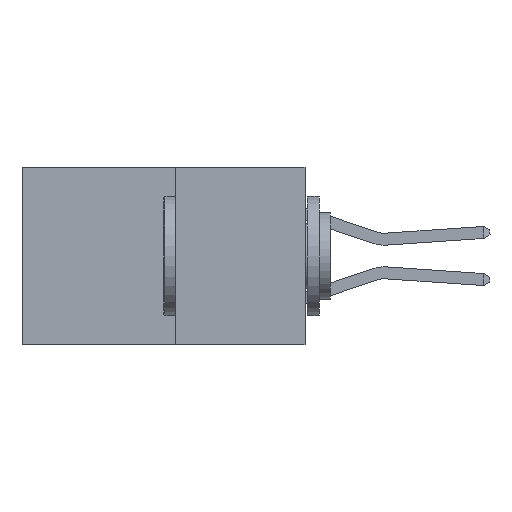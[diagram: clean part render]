
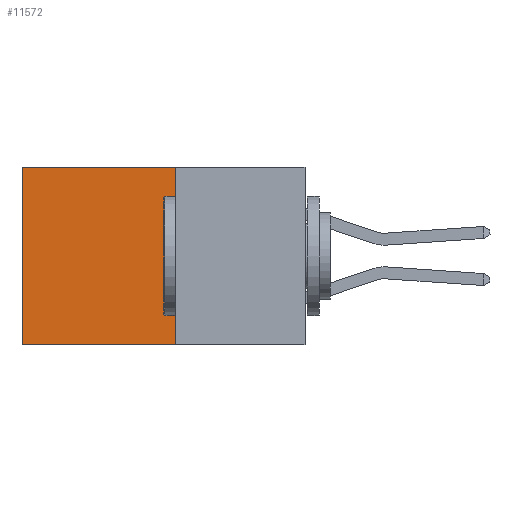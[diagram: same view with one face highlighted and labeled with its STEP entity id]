
A CAD part, left-side view. The second image highlights one B-rep face of the part: STEP entity #11572.
In plain terms, the highlighted planar face has unit normal (-1, 0, 0).
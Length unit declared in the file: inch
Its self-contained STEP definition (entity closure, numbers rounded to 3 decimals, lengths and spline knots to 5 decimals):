
#78 = VERTEX_POINT ( 'NONE', #3665 ) ;
#897 = CARTESIAN_POINT ( 'NONE',  ( 0.277, 0.27, 0. ) ) ;
#2368 = AXIS2_PLACEMENT_3D ( 'NONE', #15772, #6778, #19437 ) ;
#2902 = DIRECTION ( 'NONE',  ( 0., 0., -1. ) ) ;
#3665 = CARTESIAN_POINT ( 'NONE',  ( 0.277, 0.27, -0.37 ) ) ;
#3855 = LINE ( 'NONE', #17433, #17762 ) ;
#4111 = CARTESIAN_POINT ( 'NONE',  ( 0.277, 0.27, -0.37 ) ) ;
#4537 = CARTESIAN_POINT ( 'NONE',  ( 0.277, 0.59, -0.37 ) ) ;
#4539 = VECTOR ( 'NONE', #16781, 39.37008 ) ;
#4822 = LINE ( 'NONE', #22801, #9086 ) ;
#5117 = LINE ( 'NONE', #4111, #4539 ) ;
#6778 = DIRECTION ( 'NONE',  ( 1., 0., 0. ) ) ;
#8718 = VECTOR ( 'NONE', #19050, 39.37008 ) ;
#9086 = VECTOR ( 'NONE', #2902, 39.37008 ) ;
#9468 = EDGE_CURVE ( 'NONE', #78, #17391, #3855, .T. ) ;
#10174 = VERTEX_POINT ( 'NONE', #15640 ) ;
#11474 = VERTEX_POINT ( 'NONE', #897 ) ;
#11572 = ADVANCED_FACE ( 'NONE', ( #11981 ), #15694, .F. ) ;
#11981 = FACE_OUTER_BOUND ( 'NONE', #17147, .T. ) ;
#13414 = ORIENTED_EDGE ( 'NONE', *, *, #13504, .T. ) ;
#13504 = EDGE_CURVE ( 'NONE', #11474, #10174, #23144, .T. ) ;
#13761 = DIRECTION ( 'NONE',  ( 0., 1., 0. ) ) ;
#15530 = ORIENTED_EDGE ( 'NONE', *, *, #9468, .F. ) ;
#15640 = CARTESIAN_POINT ( 'NONE',  ( 0.277, 0.59, 0. ) ) ;
#15694 = PLANE ( 'NONE',  #2368 ) ;
#15772 = CARTESIAN_POINT ( 'NONE',  ( 0.277, 0.27, -0.37 ) ) ;
#16781 = DIRECTION ( 'NONE',  ( 0., 0., -1. ) ) ;
#17147 = EDGE_LOOP ( 'NONE', ( #18740, #15530, #20108, #13414 ) ) ;
#17391 = VERTEX_POINT ( 'NONE', #4537 ) ;
#17433 = CARTESIAN_POINT ( 'NONE',  ( 0.277, 0.27, -0.37 ) ) ;
#17762 = VECTOR ( 'NONE', #13761, 39.37008 ) ;
#17912 = EDGE_CURVE ( 'NONE', #11474, #78, #5117, .T. ) ;
#18163 = EDGE_CURVE ( 'NONE', #10174, #17391, #4822, .T. ) ;
#18740 = ORIENTED_EDGE ( 'NONE', *, *, #18163, .T. ) ;
#19050 = DIRECTION ( 'NONE',  ( 0., 1., 0. ) ) ;
#19437 = DIRECTION ( 'NONE',  ( 0., 0., -1. ) ) ;
#20108 = ORIENTED_EDGE ( 'NONE', *, *, #17912, .F. ) ;
#22671 = CARTESIAN_POINT ( 'NONE',  ( 0.277, 0.27, 0. ) ) ;
#22801 = CARTESIAN_POINT ( 'NONE',  ( 0.277, 0.59, -0.37 ) ) ;
#23144 = LINE ( 'NONE', #22671, #8718 ) ;
